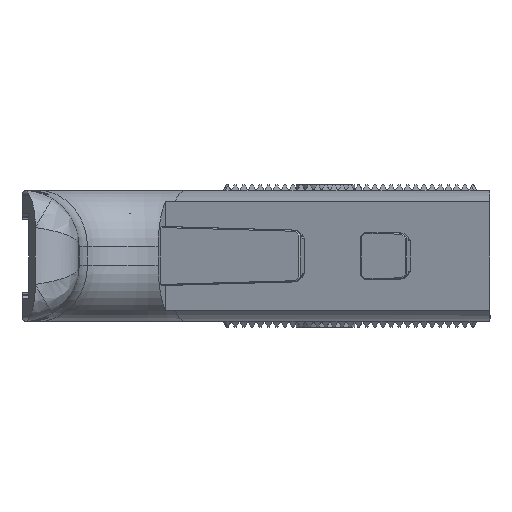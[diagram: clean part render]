
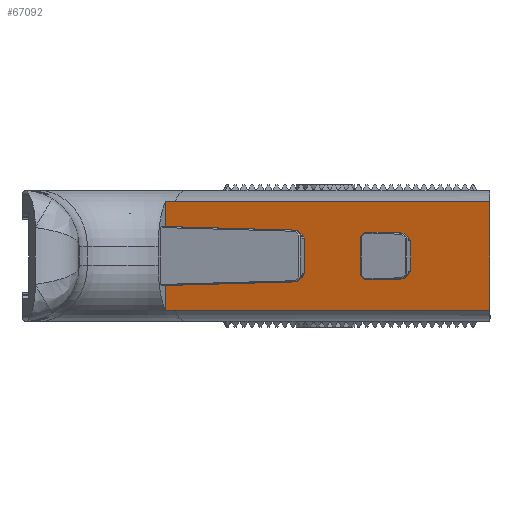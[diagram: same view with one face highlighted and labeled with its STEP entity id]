
A CAD part, left-side view. The second image highlights one B-rep face of the part: STEP entity #67092.
In plain terms, the highlighted planar face has unit normal (-0.951, 0.309, 0).
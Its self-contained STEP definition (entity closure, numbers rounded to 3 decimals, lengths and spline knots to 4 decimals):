
#231=FACE_BOUND('',#13394,.T.);
#679=B_SPLINE_CURVE_WITH_KNOTS('',3,(#121800,#121801,#121802,#121803,#121804,
#121805,#121806),.UNSPECIFIED.,.F.,.F.,(4,3,4),(0.,0.1181,0.2155),
 .UNSPECIFIED.);
#680=B_SPLINE_CURVE_WITH_KNOTS('',3,(#121814,#121815,#121816,#121817,#121818,
#121819,#121820),.UNSPECIFIED.,.F.,.F.,(4,3,4),(-0.2155,-0.1181,
0.),.UNSPECIFIED.);
#4789=PLANE('',#71440);
#9000=FACE_OUTER_BOUND('',#13393,.T.);
#13393=EDGE_LOOP('',(#60741,#60742,#60743,#60744,#60745,#60746,#60747,#60748,
#60749,#60750,#60751,#60752));
#13394=EDGE_LOOP('',(#60753,#60754,#60755,#60756,#60757,#60758,#60759,#60760,
#60761));
#21390=LINE('',#121689,#29739);
#21408=LINE('',#121727,#29757);
#21416=LINE('',#121744,#29765);
#21421=LINE('',#121753,#29770);
#21423=LINE('',#121756,#29772);
#21425=LINE('',#121761,#29774);
#21427=LINE('',#121765,#29776);
#21429=LINE('',#121768,#29778);
#21431=LINE('',#121772,#29780);
#21432=LINE('',#121774,#29781);
#21438=LINE('',#121787,#29787);
#21440=LINE('',#121791,#29789);
#21441=LINE('',#121794,#29790);
#21443=LINE('',#121798,#29792);
#21444=LINE('',#121808,#29793);
#21445=LINE('',#121810,#29794);
#21446=LINE('',#121812,#29795);
#21447=LINE('',#121822,#29796);
#21448=LINE('',#121823,#29797);
#29739=VECTOR('',#87444,0.3937);
#29757=VECTOR('',#87480,0.3937);
#29765=VECTOR('',#87494,0.3937);
#29770=VECTOR('',#87503,0.3937);
#29772=VECTOR('',#87507,0.3937);
#29774=VECTOR('',#87511,0.3937);
#29776=VECTOR('',#87515,0.3937);
#29778=VECTOR('',#87519,0.3937);
#29780=VECTOR('',#87523,0.3937);
#29781=VECTOR('',#87526,0.3937);
#29787=VECTOR('',#87542,0.3937);
#29789=VECTOR('',#87546,0.3937);
#29790=VECTOR('',#87549,0.3937);
#29792=VECTOR('',#87553,0.3937);
#29793=VECTOR('',#87554,0.3937);
#29794=VECTOR('',#87555,0.3937);
#29795=VECTOR('',#87556,0.3937);
#29796=VECTOR('',#87557,0.3937);
#29797=VECTOR('',#87558,0.3937);
#34760=VERTEX_POINT('',#121686);
#34761=VERTEX_POINT('',#121688);
#34771=VERTEX_POINT('',#121724);
#34772=VERTEX_POINT('',#121726);
#34777=VERTEX_POINT('',#121741);
#34778=VERTEX_POINT('',#121743);
#34780=VERTEX_POINT('',#121752);
#34781=VERTEX_POINT('',#121758);
#34782=VERTEX_POINT('',#121760);
#34783=VERTEX_POINT('',#121764);
#34784=VERTEX_POINT('',#121770);
#34786=VERTEX_POINT('',#121785);
#34787=VERTEX_POINT('',#121789);
#34788=VERTEX_POINT('',#121793);
#34789=VERTEX_POINT('',#121797);
#34790=VERTEX_POINT('',#121799);
#34791=VERTEX_POINT('',#121807);
#34792=VERTEX_POINT('',#121809);
#34793=VERTEX_POINT('',#121811);
#34794=VERTEX_POINT('',#121813);
#34795=VERTEX_POINT('',#121821);
#43519=EDGE_CURVE('',#34761,#34760,#21390,.T.);
#43537=EDGE_CURVE('',#34771,#34772,#21408,.T.);
#43545=EDGE_CURVE('',#34777,#34778,#21416,.F.);
#43550=EDGE_CURVE('',#34761,#34780,#21421,.F.);
#43552=EDGE_CURVE('',#34777,#34780,#21423,.T.);
#43554=EDGE_CURVE('',#34781,#34782,#21425,.F.);
#43556=EDGE_CURVE('',#34783,#34782,#21427,.T.);
#43558=EDGE_CURVE('',#34781,#34778,#21429,.T.);
#43560=EDGE_CURVE('',#34784,#34760,#21431,.F.);
#43561=EDGE_CURVE('',#34783,#34784,#21432,.F.);
#43567=EDGE_CURVE('',#34786,#34771,#21438,.F.);
#43569=EDGE_CURVE('',#34786,#34787,#21440,.T.);
#43570=EDGE_CURVE('',#34772,#34788,#21441,.F.);
#43572=EDGE_CURVE('',#34789,#34787,#21443,.T.);
#43573=EDGE_CURVE('',#34790,#34789,#679,.T.);
#43574=EDGE_CURVE('',#34791,#34790,#21444,.T.);
#43575=EDGE_CURVE('',#34792,#34791,#21445,.T.);
#43576=EDGE_CURVE('',#34793,#34792,#21446,.T.);
#43577=EDGE_CURVE('',#34794,#34793,#680,.T.);
#43578=EDGE_CURVE('',#34795,#34794,#21447,.T.);
#43579=EDGE_CURVE('',#34795,#34788,#21448,.T.);
#60741=ORIENTED_EDGE('',*,*,#43569,.T.);
#60742=ORIENTED_EDGE('',*,*,#43572,.F.);
#60743=ORIENTED_EDGE('',*,*,#43573,.F.);
#60744=ORIENTED_EDGE('',*,*,#43574,.F.);
#60745=ORIENTED_EDGE('',*,*,#43575,.F.);
#60746=ORIENTED_EDGE('',*,*,#43576,.F.);
#60747=ORIENTED_EDGE('',*,*,#43577,.F.);
#60748=ORIENTED_EDGE('',*,*,#43578,.F.);
#60749=ORIENTED_EDGE('',*,*,#43579,.T.);
#60750=ORIENTED_EDGE('',*,*,#43570,.F.);
#60751=ORIENTED_EDGE('',*,*,#43537,.F.);
#60752=ORIENTED_EDGE('',*,*,#43567,.F.);
#60753=ORIENTED_EDGE('',*,*,#43519,.T.);
#60754=ORIENTED_EDGE('',*,*,#43560,.F.);
#60755=ORIENTED_EDGE('',*,*,#43561,.F.);
#60756=ORIENTED_EDGE('',*,*,#43556,.T.);
#60757=ORIENTED_EDGE('',*,*,#43554,.F.);
#60758=ORIENTED_EDGE('',*,*,#43558,.T.);
#60759=ORIENTED_EDGE('',*,*,#43545,.F.);
#60760=ORIENTED_EDGE('',*,*,#43552,.T.);
#60761=ORIENTED_EDGE('',*,*,#43550,.F.);
#67092=ADVANCED_FACE('',(#9000,#231),#4789,.T.);
#71440=AXIS2_PLACEMENT_3D('',#121796,#87551,#87552);
#87444=DIRECTION('',(0.,0.,1.));
#87480=DIRECTION('',(0.,0.,1.));
#87494=DIRECTION('',(0.216,0.664,-0.716));
#87503=DIRECTION('',(0.221,0.681,0.698));
#87507=DIRECTION('',(0.309,0.951,-0.026));
#87511=DIRECTION('',(-0.216,-0.664,-0.716));
#87515=DIRECTION('',(-0.309,-0.951,-0.026));
#87519=DIRECTION('',(0.,0.,-1.));
#87523=DIRECTION('',(-0.12,-0.37,0.921));
#87526=DIRECTION('',(-0.221,-0.681,0.698));
#87542=DIRECTION('',(0.216,0.664,-0.716));
#87546=DIRECTION('',(0.309,0.951,-0.026));
#87549=DIRECTION('',(-0.216,-0.664,-0.716));
#87551=DIRECTION('center_axis',(-0.951,0.309,0.));
#87552=DIRECTION('ref_axis',(0.,0.,
1.));
#87553=DIRECTION('',(0.,0.,1.));
#87554=DIRECTION('',(0.309,0.951,0.));
#87555=DIRECTION('',(0.,0.,-1.));
#87556=DIRECTION('',(-0.309,-0.951,0.));
#87557=DIRECTION('',(0.,0.,1.));
#87558=DIRECTION('',(-0.309,-0.951,-0.026));
#121686=CARTESIAN_POINT('',(-2.8962,-0.8838,-0.6352));
#121688=CARTESIAN_POINT('',(-2.8962,-0.8838,-0.9101));
#121689=CARTESIAN_POINT('',(-2.8962,-0.8838,-0.7677));
#121724=CARTESIAN_POINT('',(-2.7262,-0.3607,-0.9245));
#121726=CARTESIAN_POINT('',(-2.7262,-0.3607,-0.6109));
#121727=CARTESIAN_POINT('',(-2.7262,-0.3607,-0.9154));
#121741=CARTESIAN_POINT('',(-3.0247,-1.2792,-0.909));
#121743=CARTESIAN_POINT('',(-3.0277,-1.2886,-0.8989));
#121744=CARTESIAN_POINT('',(-2.9908,-1.1749,-1.0217));
#121752=CARTESIAN_POINT('',(-2.8992,-0.8932,-0.9197));
#121753=CARTESIAN_POINT('',(-2.8709,-0.806,-0.8303));
#121756=CARTESIAN_POINT('',(-3.0469,-1.3476,-0.9072));
#121758=CARTESIAN_POINT('',(-3.0277,-1.2886,-0.6365));
#121760=CARTESIAN_POINT('',(-3.0247,-1.2792,-0.6264));
#121761=CARTESIAN_POINT('',(-2.9908,-1.1749,-0.5138));
#121764=CARTESIAN_POINT('',(-2.8992,-0.8932,-0.6158));
#121765=CARTESIAN_POINT('',(-3.0469,-1.3476,-0.6283));
#121768=CARTESIAN_POINT('',(-3.0277,-1.2886,-0.899));
#121770=CARTESIAN_POINT('',(-2.8984,-0.8905,-0.6185));
#121772=CARTESIAN_POINT('',(-2.885,-0.8493,-0.7213));
#121774=CARTESIAN_POINT('',(-2.8709,-0.806,-0.7051));
#121785=CARTESIAN_POINT('',(-2.7232,-0.3514,-0.9346));
#121787=CARTESIAN_POINT('',(-2.7647,-0.479,-0.7968));
#121789=CARTESIAN_POINT('',(-2.3324,0.8513,-0.9677));
#121791=CARTESIAN_POINT('',(-3.0469,-1.3476,-0.9072));
#121793=CARTESIAN_POINT('',(-2.7232,-0.3514,-0.6008));
#121794=CARTESIAN_POINT('',(-2.7647,-0.479,-0.7386));
#121796=CARTESIAN_POINT('Origin',(-2.8375,-0.7031,
-0.7677));
#121797=CARTESIAN_POINT('',(-2.3324,0.8513,-1.2459));
#121798=CARTESIAN_POINT('',(-2.3324,0.8513,-1.0302));
#121799=CARTESIAN_POINT('',(-2.3592,0.7689,-1.2425));
#121800=CARTESIAN_POINT('Ctrl Pts',(-2.3592,0.7689,
-1.2425));
#121801=CARTESIAN_POINT('Ctrl Pts',(-2.3544,0.7836,
-1.2425));
#121802=CARTESIAN_POINT('Ctrl Pts',(-2.3495,0.7986,
-1.2428));
#121803=CARTESIAN_POINT('Ctrl Pts',(-2.3446,0.8138,
-1.2435));
#121804=CARTESIAN_POINT('Ctrl Pts',(-2.3405,0.8264,
-1.2441));
#121805=CARTESIAN_POINT('Ctrl Pts',(-2.3365,0.8388,
-1.2449));
#121806=CARTESIAN_POINT('Ctrl Pts',(-2.3324,0.8513,
-1.2459));
#121807=CARTESIAN_POINT('',(-3.2516,-1.9775,-1.2425));
#121808=CARTESIAN_POINT('',(-2.1969,1.2684,-1.2425));
#121809=CARTESIAN_POINT('',(-3.2516,-1.9775,-0.2929));
#121810=CARTESIAN_POINT('',(-3.2516,-1.9775,-0.3839));
#121811=CARTESIAN_POINT('',(-2.3592,0.7689,-0.2929));
#121812=CARTESIAN_POINT('',(-2.6906,-0.2509,-0.2929));
#121813=CARTESIAN_POINT('',(-2.3324,0.8513,-0.2895));
#121814=CARTESIAN_POINT('Ctrl Pts',(-2.3324,0.8513,
-0.2895));
#121815=CARTESIAN_POINT('Ctrl Pts',(-2.3365,0.8388,
-0.2905));
#121816=CARTESIAN_POINT('Ctrl Pts',(-2.3405,0.8264,
-0.2913));
#121817=CARTESIAN_POINT('Ctrl Pts',(-2.3446,0.8138,
-0.2919));
#121818=CARTESIAN_POINT('Ctrl Pts',(-2.3495,0.7986,
-0.2926));
#121819=CARTESIAN_POINT('Ctrl Pts',(-2.3544,0.7836,
-0.2929));
#121820=CARTESIAN_POINT('Ctrl Pts',(-2.3592,0.7689,
-0.2929));
#121821=CARTESIAN_POINT('',(-2.3324,0.8513,-0.5677));
#121822=CARTESIAN_POINT('',(-2.3324,0.8513,-0.7677));
#121823=CARTESIAN_POINT('',(-3.0469,-1.3476,-0.6283));
